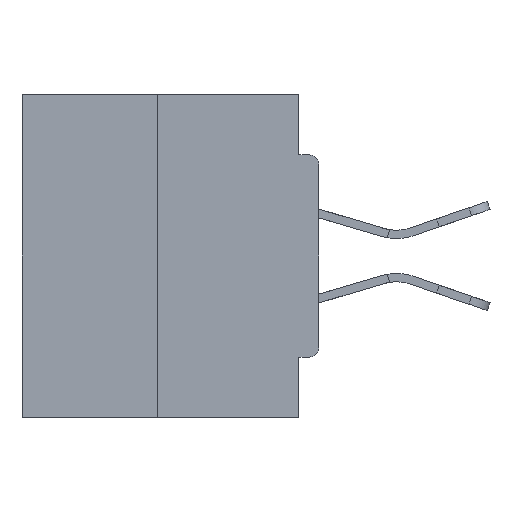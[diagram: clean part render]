
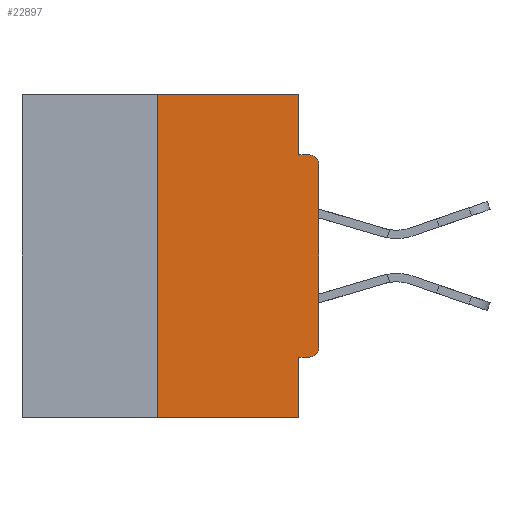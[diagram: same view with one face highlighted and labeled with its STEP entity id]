
A CAD part, left-side view. The second image highlights one B-rep face of the part: STEP entity #22897.
In plain terms, the highlighted planar face has unit normal (-1, 0, 0).
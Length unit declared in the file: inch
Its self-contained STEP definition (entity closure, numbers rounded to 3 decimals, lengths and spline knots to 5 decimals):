
#391 = LINE ( 'NONE', #26045, #1717 ) ;
#875 = CARTESIAN_POINT ( 'NONE',  ( 0., 0.46, -0.5 ) ) ;
#1042 = EDGE_CURVE ( 'NONE', #34962, #29479, #391, .T. ) ;
#1717 = VECTOR ( 'NONE', #12213, 39.37008 ) ;
#2748 = VECTOR ( 'NONE', #25362, 39.37008 ) ;
#3647 = LINE ( 'NONE', #8203, #2748 ) ;
#3678 = CARTESIAN_POINT ( 'NONE',  ( 0., 0.031, 0. ) ) ;
#3925 = DIRECTION ( 'NONE',  ( 0., -1., 0. ) ) ;
#4530 = DIRECTION ( 'NONE',  ( 0., 0., -1. ) ) ;
#4611 = EDGE_LOOP ( 'NONE', ( #8492, #31478, #9363, #16397, #29445, #20808, #23797, #18935, #14395, #13610 ) ) ;
#4904 = DIRECTION ( 'NONE',  ( 0., 0., 1. ) ) ;
#5248 = VERTEX_POINT ( 'NONE', #26700 ) ;
#6054 = CARTESIAN_POINT ( 'NONE',  ( 0., 0.015, -0.0935 ) ) ;
#6143 = EDGE_CURVE ( 'NONE', #10043, #32413, #3647, .T. ) ;
#6296 = AXIS2_PLACEMENT_3D ( 'NONE', #31445, #23340, #12220 ) ;
#7588 = VERTEX_POINT ( 'NONE', #15252 ) ;
#8203 = CARTESIAN_POINT ( 'NONE',  ( 0., 0., 0. ) ) ;
#8492 = ORIENTED_EDGE ( 'NONE', *, *, #11969, .F. ) ;
#9085 = CARTESIAN_POINT ( 'NONE',  ( 0., 0.25, 0. ) ) ;
#9309 = DIRECTION ( 'NONE',  ( 0., -1., 0. ) ) ;
#9363 = ORIENTED_EDGE ( 'NONE', *, *, #14402, .T. ) ;
#9377 = CARTESIAN_POINT ( 'NONE',  ( 0., 0.25, -0.5 ) ) ;
#9418 = FACE_OUTER_BOUND ( 'NONE', #4611, .T. ) ;
#9886 = VECTOR ( 'NONE', #3925, 39.37008 ) ;
#9958 = AXIS2_PLACEMENT_3D ( 'NONE', #35148, #18553, #4530 ) ;
#10043 = VERTEX_POINT ( 'NONE', #36006 ) ;
#10674 = CARTESIAN_POINT ( 'NONE',  ( 0., 0., -0.1085 ) ) ;
#11969 = EDGE_CURVE ( 'NONE', #29393, #34962, #29593, .T. ) ;
#12154 = VERTEX_POINT ( 'NONE', #30562 ) ;
#12213 = DIRECTION ( 'NONE',  ( 0., 0., -1. ) ) ;
#12220 = DIRECTION ( 'NONE',  ( 0., 0., -1. ) ) ;
#12597 = VECTOR ( 'NONE', #14433, 39.37008 ) ;
#13354 = CARTESIAN_POINT ( 'NONE',  ( 0., 0.015, -0.3915 ) ) ;
#13610 = ORIENTED_EDGE ( 'NONE', *, *, #1042, .F. ) ;
#13948 = EDGE_CURVE ( 'NONE', #26802, #29393, #19812, .T. ) ;
#14395 = ORIENTED_EDGE ( 'NONE', *, *, #34634, .F. ) ;
#14402 = EDGE_CURVE ( 'NONE', #26802, #12154, #30358, .T. ) ;
#14433 = DIRECTION ( 'NONE',  ( 0., 0., -1. ) ) ;
#14609 = EDGE_CURVE ( 'NONE', #32413, #31551, #20192, .T. ) ;
#15252 = CARTESIAN_POINT ( 'NONE',  ( 0., 0.031, -0.4065 ) ) ;
#16397 = ORIENTED_EDGE ( 'NONE', *, *, #28514, .F. ) ;
#17946 = CARTESIAN_POINT ( 'NONE',  ( 0., 0.46, 0. ) ) ;
#18553 = DIRECTION ( 'NONE',  ( -1., 0., 0. ) ) ;
#18935 = ORIENTED_EDGE ( 'NONE', *, *, #14609, .T. ) ;
#18983 = DIRECTION ( 'NONE',  ( 0., 0., -1. ) ) ;
#19812 = LINE ( 'NONE', #27244, #23344 ) ;
#20192 = CIRCLE ( 'NONE', #9958, 0.015 ) ;
#20808 = ORIENTED_EDGE ( 'NONE', *, *, #25894, .T. ) ;
#22897 = ADVANCED_FACE ( 'NONE', ( #9418 ), #25803, .F. ) ;
#23340 = DIRECTION ( 'NONE',  ( 1., 0., 0. ) ) ;
#23344 = VECTOR ( 'NONE', #4904, 39.37008 ) ;
#23797 = ORIENTED_EDGE ( 'NONE', *, *, #6143, .T. ) ;
#25090 = DIRECTION ( 'NONE',  ( 0., -1., 0. ) ) ;
#25328 = CARTESIAN_POINT ( 'NONE',  ( 0., 0., -0.0935 ) ) ;
#25362 = DIRECTION ( 'NONE',  ( 0., 0., 1. ) ) ;
#25803 = PLANE ( 'NONE',  #6296 ) ;
#25894 = EDGE_CURVE ( 'NONE', #5248, #10043, #34799, .T. ) ;
#26045 = CARTESIAN_POINT ( 'NONE',  ( 0., 0.031, 0. ) ) ;
#26700 = CARTESIAN_POINT ( 'NONE',  ( 0., 0.015, -0.4065 ) ) ;
#26714 = LINE ( 'NONE', #25328, #30638 ) ;
#26802 = VERTEX_POINT ( 'NONE', #9377 ) ;
#27244 = CARTESIAN_POINT ( 'NONE',  ( 0., 0.25, 0. ) ) ;
#27332 = AXIS2_PLACEMENT_3D ( 'NONE', #13354, #35853, #18983 ) ;
#27502 = LINE ( 'NONE', #33958, #12597 ) ;
#28021 = CARTESIAN_POINT ( 'NONE',  ( 0., 0.031, -0.0935 ) ) ;
#28514 = EDGE_CURVE ( 'NONE', #7588, #12154, #27502, .T. ) ;
#29393 = VERTEX_POINT ( 'NONE', #9085 ) ;
#29445 = ORIENTED_EDGE ( 'NONE', *, *, #34252, .F. ) ;
#29479 = VERTEX_POINT ( 'NONE', #28021 ) ;
#29593 = LINE ( 'NONE', #17946, #9886 ) ;
#30358 = LINE ( 'NONE', #875, #30782 ) ;
#30562 = CARTESIAN_POINT ( 'NONE',  ( 0., 0.031, -0.5 ) ) ;
#30638 = VECTOR ( 'NONE', #25090, 39.37008 ) ;
#30782 = VECTOR ( 'NONE', #9309, 39.37008 ) ;
#31445 = CARTESIAN_POINT ( 'NONE',  ( 0., 0.46, 0. ) ) ;
#31478 = ORIENTED_EDGE ( 'NONE', *, *, #13948, .F. ) ;
#31497 = DIRECTION ( 'NONE',  ( 0., 1., 0. ) ) ;
#31551 = VERTEX_POINT ( 'NONE', #6054 ) ;
#32413 = VERTEX_POINT ( 'NONE', #10674 ) ;
#33265 = VECTOR ( 'NONE', #31497, 39.37008 ) ;
#33958 = CARTESIAN_POINT ( 'NONE',  ( 0., 0.031, -0.5 ) ) ;
#34252 = EDGE_CURVE ( 'NONE', #5248, #7588, #35044, .T. ) ;
#34634 = EDGE_CURVE ( 'NONE', #29479, #31551, #26714, .T. ) ;
#34799 = CIRCLE ( 'NONE', #27332, 0.015 ) ;
#34962 = VERTEX_POINT ( 'NONE', #3678 ) ;
#35044 = LINE ( 'NONE', #36209, #33265 ) ;
#35148 = CARTESIAN_POINT ( 'NONE',  ( 0., 0.015, -0.1085 ) ) ;
#35853 = DIRECTION ( 'NONE',  ( -1., 0., 0. ) ) ;
#36006 = CARTESIAN_POINT ( 'NONE',  ( 0., 0., -0.3915 ) ) ;
#36209 = CARTESIAN_POINT ( 'NONE',  ( 0., 0., -0.4065 ) ) ;
